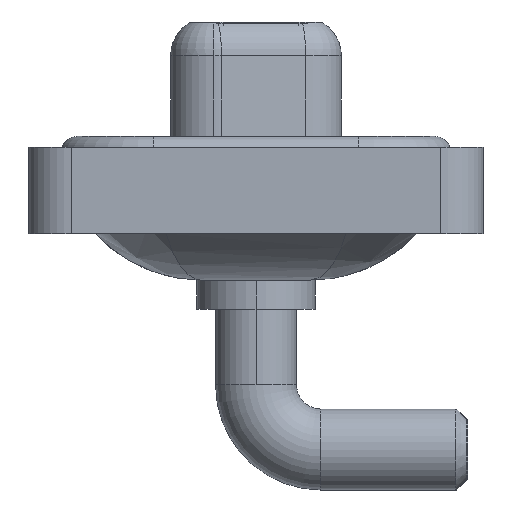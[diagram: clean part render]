
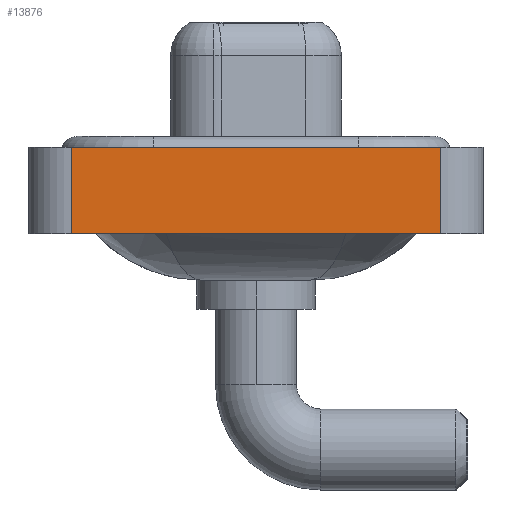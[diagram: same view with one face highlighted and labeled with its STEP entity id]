
A CAD part, left-side view. The second image highlights one B-rep face of the part: STEP entity #13876.
In plain terms, the highlighted planar face has unit normal (-1, 0, 0).
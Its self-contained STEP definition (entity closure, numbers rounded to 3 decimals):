
#60 = DIRECTION ( 'NONE',  ( -1., 0., 0. ) ) ;
#294 = EDGE_CURVE ( 'NONE', #9007, #10162, #16239, .T. ) ;
#403 = CARTESIAN_POINT ( 'NONE',  ( -7.25, -8.55, -3.6 ) ) ;
#448 = CARTESIAN_POINT ( 'NONE',  ( -7.25, -8.55, -3.6 ) ) ;
#783 = CARTESIAN_POINT ( 'NONE',  ( -7.25, -8.55, -3.6 ) ) ;
#1219 = CARTESIAN_POINT ( 'NONE',  ( -7.25, -8.55, 0.4 ) ) ;
#1245 = ORIENTED_EDGE ( 'NONE', *, *, #7241, .T. ) ;
#1419 = CARTESIAN_POINT ( 'NONE',  ( -7.25, 8.55, 0.4 ) ) ;
#1607 = ORIENTED_EDGE ( 'NONE', *, *, #14251, .F. ) ;
#2264 = VECTOR ( 'NONE', #10351, 1000. ) ;
#2596 = ORIENTED_EDGE ( 'NONE', *, *, #4989, .F. ) ;
#2735 = VECTOR ( 'NONE', #8853, 1000. ) ;
#3026 = VERTEX_POINT ( 'NONE', #12137 ) ;
#4293 = VERTEX_POINT ( 'NONE', #1419 ) ;
#4989 = EDGE_CURVE ( 'NONE', #9007, #4293, #12969, .T. ) ;
#5020 = LINE ( 'NONE', #1219, #2264 ) ;
#5718 = CARTESIAN_POINT ( 'NONE',  ( -7.25, -8.55, -3.6 ) ) ;
#6191 = CARTESIAN_POINT ( 'NONE',  ( -7.25, 8.55, -3.6 ) ) ;
#7241 = EDGE_CURVE ( 'NONE', #10162, #3026, #15219, .T. ) ;
#8451 = DIRECTION ( 'NONE',  ( 0., -1., 0. ) ) ;
#8853 = DIRECTION ( 'NONE',  ( 0., 0., 1. ) ) ;
#9007 = VERTEX_POINT ( 'NONE', #15730 ) ;
#9343 = AXIS2_PLACEMENT_3D ( 'NONE', #403, #60, #10472 ) ;
#9473 = EDGE_LOOP ( 'NONE', ( #1245, #1607, #2596, #13351 ) ) ;
#10162 = VERTEX_POINT ( 'NONE', #448 ) ;
#10351 = DIRECTION ( 'NONE',  ( 0., -1., 0. ) ) ;
#10472 = DIRECTION ( 'NONE',  ( 0., 0., 1. ) ) ;
#12009 = PLANE ( 'NONE',  #9343 ) ;
#12137 = CARTESIAN_POINT ( 'NONE',  ( -7.25, -8.55, 0.4 ) ) ;
#12969 = LINE ( 'NONE', #6191, #2735 ) ;
#13351 = ORIENTED_EDGE ( 'NONE', *, *, #294, .T. ) ;
#13876 = ADVANCED_FACE ( 'NONE', ( #15775 ), #12009, .T. ) ;
#14251 = EDGE_CURVE ( 'NONE', #4293, #3026, #5020, .T. ) ;
#15219 = LINE ( 'NONE', #5718, #16511 ) ;
#15730 = CARTESIAN_POINT ( 'NONE',  ( -7.25, 8.55, -3.6 ) ) ;
#15775 = FACE_OUTER_BOUND ( 'NONE', #9473, .T. ) ;
#16173 = DIRECTION ( 'NONE',  ( 0., 0., 1. ) ) ;
#16239 = LINE ( 'NONE', #783, #16262 ) ;
#16262 = VECTOR ( 'NONE', #8451, 1000. ) ;
#16511 = VECTOR ( 'NONE', #16173, 1000. ) ;
